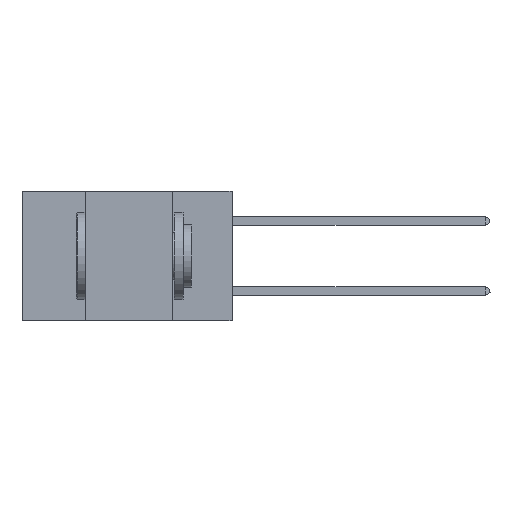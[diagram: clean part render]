
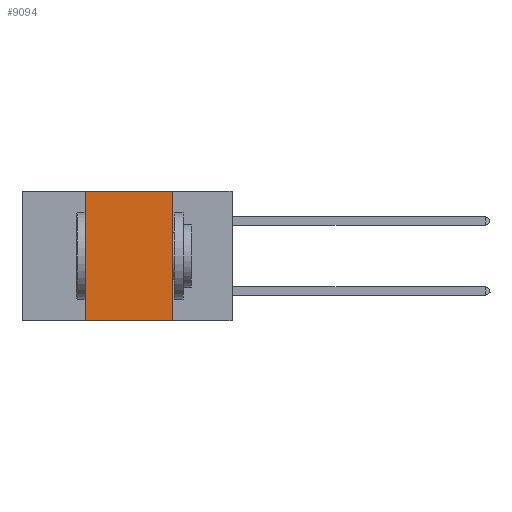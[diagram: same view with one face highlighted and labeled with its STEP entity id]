
A CAD part, left-side view. The second image highlights one B-rep face of the part: STEP entity #9094.
In plain terms, the highlighted planar face has unit normal (-1, 0, 0).
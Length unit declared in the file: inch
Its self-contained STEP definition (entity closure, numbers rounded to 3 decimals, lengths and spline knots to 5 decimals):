
#319 = VERTEX_POINT ( 'NONE', #26109 ) ;
#1259 = VECTOR ( 'NONE', #28394, 39.37008 ) ;
#1648 = EDGE_LOOP ( 'NONE', ( #5073, #26642, #12370, #28564 ) ) ;
#1838 = LINE ( 'NONE', #10892, #11856 ) ;
#2062 = CARTESIAN_POINT ( 'NONE',  ( 0., 0.6, 0. ) ) ;
#2852 = CARTESIAN_POINT ( 'NONE',  ( 0., 0.42, 0. ) ) ;
#2948 = CARTESIAN_POINT ( 'NONE',  ( 0., 0.17, -0.37 ) ) ;
#4596 = VERTEX_POINT ( 'NONE', #2948 ) ;
#5073 = ORIENTED_EDGE ( 'NONE', *, *, #12576, .F. ) ;
#6119 = CARTESIAN_POINT ( 'NONE',  ( 0., 0.42, -0.37 ) ) ;
#7675 = EDGE_CURVE ( 'NONE', #11350, #4596, #1838, .T. ) ;
#9094 = ADVANCED_FACE ( 'NONE', ( #22953 ), #17940, .F. ) ;
#10892 = CARTESIAN_POINT ( 'NONE',  ( 0., 0.6, -0.37 ) ) ;
#11350 = VERTEX_POINT ( 'NONE', #6119 ) ;
#11856 = VECTOR ( 'NONE', #15500, 39.37008 ) ;
#12152 = DIRECTION ( 'NONE',  ( 0., 0., 1. ) ) ;
#12370 = ORIENTED_EDGE ( 'NONE', *, *, #16819, .F. ) ;
#12576 = EDGE_CURVE ( 'NONE', #319, #4596, #14130, .T. ) ;
#13247 = VERTEX_POINT ( 'NONE', #19385 ) ;
#14130 = LINE ( 'NONE', #28290, #1259 ) ;
#14347 = CARTESIAN_POINT ( 'NONE',  ( 0., 0.6, 0. ) ) ;
#14348 = AXIS2_PLACEMENT_3D ( 'NONE', #2062, #27285, #17835 ) ;
#15500 = DIRECTION ( 'NONE',  ( 0., -1., 0. ) ) ;
#16819 = EDGE_CURVE ( 'NONE', #11350, #13247, #17784, .T. ) ;
#17784 = LINE ( 'NONE', #2852, #21011 ) ;
#17835 = DIRECTION ( 'NONE',  ( 0., 0., -1. ) ) ;
#17940 = PLANE ( 'NONE',  #14348 ) ;
#19385 = CARTESIAN_POINT ( 'NONE',  ( 0., 0.42, 0. ) ) ;
#21011 = VECTOR ( 'NONE', #12152, 39.37008 ) ;
#22953 = FACE_OUTER_BOUND ( 'NONE', #1648, .T. ) ;
#24578 = VECTOR ( 'NONE', #28208, 39.37008 ) ;
#25818 = EDGE_CURVE ( 'NONE', #13247, #319, #25991, .T. ) ;
#25991 = LINE ( 'NONE', #14347, #24578 ) ;
#26109 = CARTESIAN_POINT ( 'NONE',  ( 0., 0.17, 0. ) ) ;
#26642 = ORIENTED_EDGE ( 'NONE', *, *, #25818, .F. ) ;
#27285 = DIRECTION ( 'NONE',  ( 1., 0., 0. ) ) ;
#28208 = DIRECTION ( 'NONE',  ( 0., -1., 0. ) ) ;
#28290 = CARTESIAN_POINT ( 'NONE',  ( 0., 0.17, 0. ) ) ;
#28394 = DIRECTION ( 'NONE',  ( 0., 0., -1. ) ) ;
#28564 = ORIENTED_EDGE ( 'NONE', *, *, #7675, .T. ) ;
